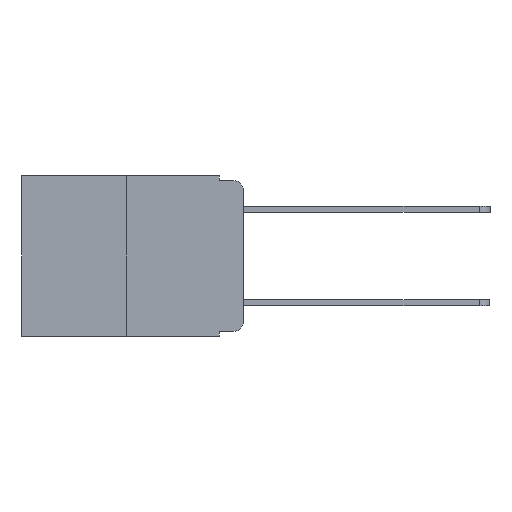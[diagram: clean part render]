
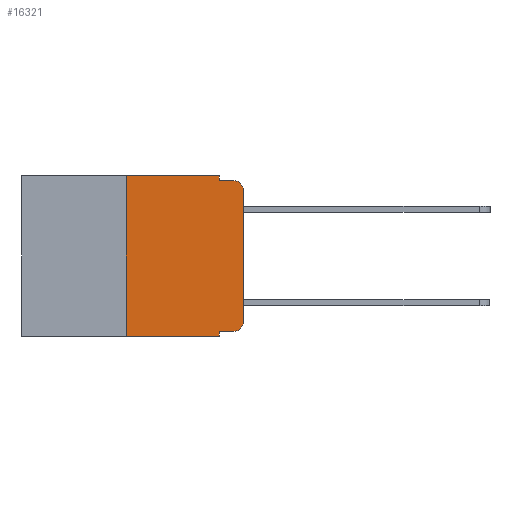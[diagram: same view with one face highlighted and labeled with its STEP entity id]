
A CAD part, left-side view. The second image highlights one B-rep face of the part: STEP entity #16321.
In plain terms, the highlighted planar face has unit normal (-1, 0, 0).
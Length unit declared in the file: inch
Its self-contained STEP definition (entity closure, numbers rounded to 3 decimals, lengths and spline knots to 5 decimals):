
#177 = EDGE_CURVE ( 'NONE', #1126, #1111, #6708, .T. ) ;
#529 = CARTESIAN_POINT ( 'NONE',  ( 0., 0.02, -0.01 ) ) ;
#535 = CARTESIAN_POINT ( 'NONE',  ( 0., 0.473, 0. ) ) ;
#705 = EDGE_CURVE ( 'NONE', #9898, #12062, #6273, .T. ) ;
#925 = AXIS2_PLACEMENT_3D ( 'NONE', #6172, #15454, #7514 ) ;
#1111 = VERTEX_POINT ( 'NONE', #15864 ) ;
#1126 = VERTEX_POINT ( 'NONE', #9180 ) ;
#1262 = VERTEX_POINT ( 'NONE', #9267 ) ;
#1800 = CARTESIAN_POINT ( 'NONE',  ( 0., 0., -0.03 ) ) ;
#1901 = CARTESIAN_POINT ( 'NONE',  ( 0., 0.051, -0.333 ) ) ;
#2162 = VECTOR ( 'NONE', #14556, 39.37008 ) ;
#2348 = EDGE_LOOP ( 'NONE', ( #2646, #2486, #6422, #8445, #16250, #16450, #9881, #8138, #8342, #9525 ) ) ;
#2401 = DIRECTION ( 'NONE',  ( 1., 0., 0. ) ) ;
#2486 = ORIENTED_EDGE ( 'NONE', *, *, #17381, .T. ) ;
#2646 = ORIENTED_EDGE ( 'NONE', *, *, #14827, .T. ) ;
#2738 = CARTESIAN_POINT ( 'NONE',  ( 0., 0.473, -0.343 ) ) ;
#2914 = LINE ( 'NONE', #4959, #6148 ) ;
#4320 = VERTEX_POINT ( 'NONE', #529 ) ;
#4647 = EDGE_CURVE ( 'NONE', #9316, #4320, #14480, .T. ) ;
#4724 = VECTOR ( 'NONE', #15040, 39.37008 ) ;
#4959 = CARTESIAN_POINT ( 'NONE',  ( 0., 0.051, 0. ) ) ;
#5114 = CARTESIAN_POINT ( 'NONE',  ( 0., 0.051, 0. ) ) ;
#5613 = CARTESIAN_POINT ( 'NONE',  ( 0., 0., 0. ) ) ;
#5819 = VERTEX_POINT ( 'NONE', #1800 ) ;
#5892 = LINE ( 'NONE', #6434, #16453 ) ;
#5924 = VERTEX_POINT ( 'NONE', #15401 ) ;
#6148 = VECTOR ( 'NONE', #15597, 39.37008 ) ;
#6172 = CARTESIAN_POINT ( 'NONE',  ( 0., 0.02, -0.03 ) ) ;
#6273 = LINE ( 'NONE', #535, #2162 ) ;
#6422 = ORIENTED_EDGE ( 'NONE', *, *, #4647, .F. ) ;
#6434 = CARTESIAN_POINT ( 'NONE',  ( 0., 0.051, 0. ) ) ;
#6608 = EDGE_CURVE ( 'NONE', #5924, #1262, #17012, .T. ) ;
#6708 = CIRCLE ( 'NONE', #8902, 0.02 ) ;
#7253 = VERTEX_POINT ( 'NONE', #10883 ) ;
#7364 = CIRCLE ( 'NONE', #925, 0.02 ) ;
#7514 = DIRECTION ( 'NONE',  ( 0., 0., -1. ) ) ;
#7813 = VECTOR ( 'NONE', #14215, 39.37008 ) ;
#7840 = PLANE ( 'NONE',  #11469 ) ;
#8138 = ORIENTED_EDGE ( 'NONE', *, *, #16213, .F. ) ;
#8342 = ORIENTED_EDGE ( 'NONE', *, *, #15045, .T. ) ;
#8399 = CARTESIAN_POINT ( 'NONE',  ( 0., 0.02, -0.313 ) ) ;
#8444 = FACE_OUTER_BOUND ( 'NONE', #2348, .T. ) ;
#8445 = ORIENTED_EDGE ( 'NONE', *, *, #10101, .F. ) ;
#8494 = VECTOR ( 'NONE', #11411, 39.37008 ) ;
#8733 = CARTESIAN_POINT ( 'NONE',  ( 0., 0.25, 0. ) ) ;
#8902 = AXIS2_PLACEMENT_3D ( 'NONE', #8399, #13401, #12184 ) ;
#9180 = CARTESIAN_POINT ( 'NONE',  ( 0., 0.02, -0.333 ) ) ;
#9267 = CARTESIAN_POINT ( 'NONE',  ( 0., 0.051, -0.343 ) ) ;
#9316 = VERTEX_POINT ( 'NONE', #12955 ) ;
#9525 = ORIENTED_EDGE ( 'NONE', *, *, #177, .T. ) ;
#9569 = DIRECTION ( 'NONE',  ( 0., -1., 0. ) ) ;
#9813 = CARTESIAN_POINT ( 'NONE',  ( 0., 0.25, 0. ) ) ;
#9881 = ORIENTED_EDGE ( 'NONE', *, *, #6608, .T. ) ;
#9898 = VERTEX_POINT ( 'NONE', #8733 ) ;
#10101 = EDGE_CURVE ( 'NONE', #12062, #9316, #5892, .T. ) ;
#10587 = CARTESIAN_POINT ( 'NONE',  ( 0., 0.473, 0. ) ) ;
#10883 = CARTESIAN_POINT ( 'NONE',  ( 0., 0.051, -0.333 ) ) ;
#11411 = DIRECTION ( 'NONE',  ( 0., -1., 0. ) ) ;
#11469 = AXIS2_PLACEMENT_3D ( 'NONE', #10587, #2401, #11934 ) ;
#11934 = DIRECTION ( 'NONE',  ( 0., 0., -1. ) ) ;
#12062 = VERTEX_POINT ( 'NONE', #5114 ) ;
#12184 = DIRECTION ( 'NONE',  ( 0., 0., -1. ) ) ;
#12537 = LINE ( 'NONE', #1901, #8494 ) ;
#12938 = CARTESIAN_POINT ( 'NONE',  ( 0., 0.051, -0.01 ) ) ;
#12955 = CARTESIAN_POINT ( 'NONE',  ( 0., 0.051, -0.01 ) ) ;
#13226 = VECTOR ( 'NONE', #9569, 39.37008 ) ;
#13401 = DIRECTION ( 'NONE',  ( -1., 0., 0. ) ) ;
#13524 = VECTOR ( 'NONE', #13670, 39.37008 ) ;
#13660 = EDGE_CURVE ( 'NONE', #5924, #9898, #14951, .T. ) ;
#13670 = DIRECTION ( 'NONE',  ( 0., 0., 1. ) ) ;
#14215 = DIRECTION ( 'NONE',  ( 0., -1., 0. ) ) ;
#14480 = LINE ( 'NONE', #12938, #7813 ) ;
#14556 = DIRECTION ( 'NONE',  ( 0., -1., 0. ) ) ;
#14827 = EDGE_CURVE ( 'NONE', #1111, #5819, #16912, .T. ) ;
#14951 = LINE ( 'NONE', #9813, #4724 ) ;
#15040 = DIRECTION ( 'NONE',  ( 0., 0., 1. ) ) ;
#15045 = EDGE_CURVE ( 'NONE', #7253, #1126, #12537, .T. ) ;
#15401 = CARTESIAN_POINT ( 'NONE',  ( 0., 0.25, -0.343 ) ) ;
#15454 = DIRECTION ( 'NONE',  ( -1., 0., 0. ) ) ;
#15597 = DIRECTION ( 'NONE',  ( 0., 0., -1. ) ) ;
#15712 = DIRECTION ( 'NONE',  ( 0., 0., -1. ) ) ;
#15864 = CARTESIAN_POINT ( 'NONE',  ( 0., 0., -0.313 ) ) ;
#16213 = EDGE_CURVE ( 'NONE', #7253, #1262, #2914, .T. ) ;
#16250 = ORIENTED_EDGE ( 'NONE', *, *, #705, .F. ) ;
#16321 = ADVANCED_FACE ( 'NONE', ( #8444 ), #7840, .F. ) ;
#16450 = ORIENTED_EDGE ( 'NONE', *, *, #13660, .F. ) ;
#16453 = VECTOR ( 'NONE', #15712, 39.37008 ) ;
#16912 = LINE ( 'NONE', #5613, #13524 ) ;
#17012 = LINE ( 'NONE', #2738, #13226 ) ;
#17381 = EDGE_CURVE ( 'NONE', #5819, #4320, #7364, .T. ) ;
